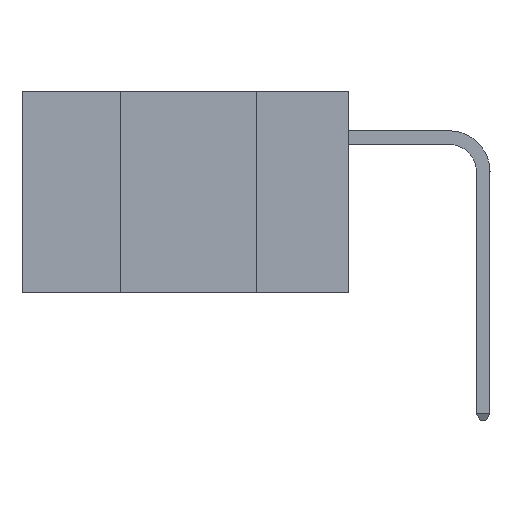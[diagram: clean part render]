
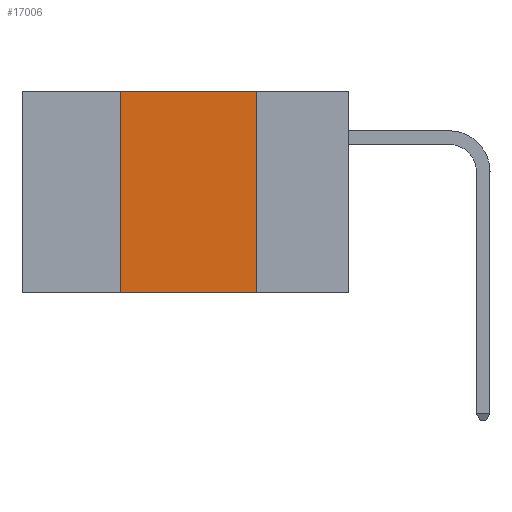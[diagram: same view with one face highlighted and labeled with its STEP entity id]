
A CAD part, left-side view. The second image highlights one B-rep face of the part: STEP entity #17006.
In plain terms, the highlighted planar face has unit normal (-1, 0, 0).
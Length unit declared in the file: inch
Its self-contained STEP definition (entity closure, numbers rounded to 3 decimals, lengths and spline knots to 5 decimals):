
#146 = CARTESIAN_POINT ( 'NONE',  ( 0., 0.42, 0. ) ) ;
#1556 = CARTESIAN_POINT ( 'NONE',  ( 0., 0.6, 0. ) ) ;
#1913 = DIRECTION ( 'NONE',  ( 0., 0., 1. ) ) ;
#1924 = ORIENTED_EDGE ( 'NONE', *, *, #4609, .T. ) ;
#2814 = VECTOR ( 'NONE', #4568, 39.37008 ) ;
#3170 = EDGE_CURVE ( 'NONE', #18988, #5342, #20159, .T. ) ;
#3248 = DIRECTION ( 'NONE',  ( 0., 0., -1. ) ) ;
#3798 = LINE ( 'NONE', #146, #12964 ) ;
#4561 = CARTESIAN_POINT ( 'NONE',  ( 0., 0.6, 0. ) ) ;
#4568 = DIRECTION ( 'NONE',  ( 0., -1., 0. ) ) ;
#4609 = EDGE_CURVE ( 'NONE', #19623, #16258, #19850, .T. ) ;
#5053 = AXIS2_PLACEMENT_3D ( 'NONE', #1556, #12981, #3248 ) ;
#5212 = FACE_OUTER_BOUND ( 'NONE', #19071, .T. ) ;
#5272 = CARTESIAN_POINT ( 'NONE',  ( 0., 0.17, 0. ) ) ;
#5342 = VERTEX_POINT ( 'NONE', #18457 ) ;
#6842 = VECTOR ( 'NONE', #19450, 39.37008 ) ;
#9137 = CARTESIAN_POINT ( 'NONE',  ( 0., 0.17, -0.37 ) ) ;
#10109 = EDGE_CURVE ( 'NONE', #19623, #18988, #3798, .T. ) ;
#11393 = PLANE ( 'NONE',  #5053 ) ;
#11589 = CARTESIAN_POINT ( 'NONE',  ( 0., 0.42, 0. ) ) ;
#11676 = VECTOR ( 'NONE', #13722, 39.37008 ) ;
#12209 = EDGE_CURVE ( 'NONE', #5342, #16258, #19308, .T. ) ;
#12407 = ORIENTED_EDGE ( 'NONE', *, *, #10109, .F. ) ;
#12568 = CARTESIAN_POINT ( 'NONE',  ( 0., 0.42, -0.37 ) ) ;
#12964 = VECTOR ( 'NONE', #1913, 39.37008 ) ;
#12981 = DIRECTION ( 'NONE',  ( 1., 0., 0. ) ) ;
#13063 = CARTESIAN_POINT ( 'NONE',  ( 0., 0.6, -0.37 ) ) ;
#13722 = DIRECTION ( 'NONE',  ( 0., -1., 0. ) ) ;
#16196 = ORIENTED_EDGE ( 'NONE', *, *, #12209, .F. ) ;
#16258 = VERTEX_POINT ( 'NONE', #9137 ) ;
#17006 = ADVANCED_FACE ( 'NONE', ( #5212 ), #11393, .F. ) ;
#18227 = ORIENTED_EDGE ( 'NONE', *, *, #3170, .F. ) ;
#18457 = CARTESIAN_POINT ( 'NONE',  ( 0., 0.17, 0. ) ) ;
#18988 = VERTEX_POINT ( 'NONE', #11589 ) ;
#19071 = EDGE_LOOP ( 'NONE', ( #16196, #18227, #12407, #1924 ) ) ;
#19308 = LINE ( 'NONE', #5272, #6842 ) ;
#19450 = DIRECTION ( 'NONE',  ( 0., 0., -1. ) ) ;
#19623 = VERTEX_POINT ( 'NONE', #12568 ) ;
#19850 = LINE ( 'NONE', #13063, #11676 ) ;
#20159 = LINE ( 'NONE', #4561, #2814 ) ;
